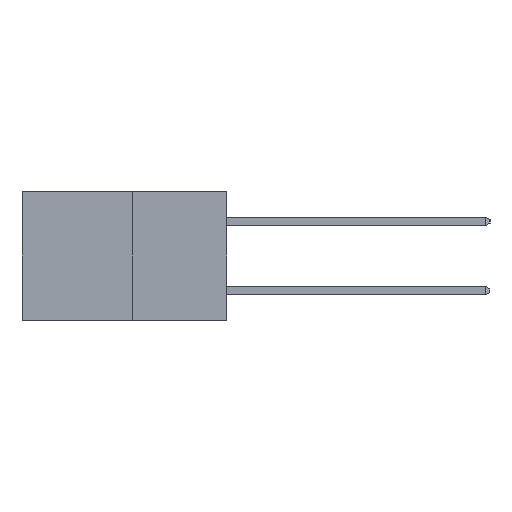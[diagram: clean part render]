
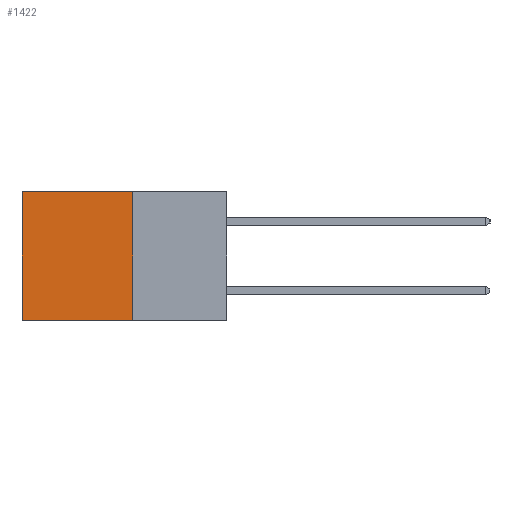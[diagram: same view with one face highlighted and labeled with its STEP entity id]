
A CAD part, left-side view. The second image highlights one B-rep face of the part: STEP entity #1422.
In plain terms, the highlighted planar face has unit normal (-1, 0, 0).
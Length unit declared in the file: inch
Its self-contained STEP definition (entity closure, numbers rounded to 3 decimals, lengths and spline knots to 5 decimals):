
#739 = DIRECTION ( 'NONE',  ( 0., 1., 0. ) ) ;
#784 = AXIS2_PLACEMENT_3D ( 'NONE', #6101, #7769, #3082 ) ;
#793 = CARTESIAN_POINT ( 'NONE',  ( 0.277, 0.59, -0.37 ) ) ;
#1271 = DIRECTION ( 'NONE',  ( 0., 1., 0. ) ) ;
#1422 = ADVANCED_FACE ( 'NONE', ( #7081 ), #3141, .F. ) ;
#1461 = DIRECTION ( 'NONE',  ( 0., 0., -1. ) ) ;
#1552 = CARTESIAN_POINT ( 'NONE',  ( 0.277, 0.27, -0.37 ) ) ;
#2052 = DIRECTION ( 'NONE',  ( 0., 0., -1. ) ) ;
#2088 = CARTESIAN_POINT ( 'NONE',  ( 0.277, 0.59, -0.37 ) ) ;
#2258 = CARTESIAN_POINT ( 'NONE',  ( 0.277, 0.27, 0. ) ) ;
#2461 = VERTEX_POINT ( 'NONE', #7559 ) ;
#2623 = VERTEX_POINT ( 'NONE', #793 ) ;
#2718 = VERTEX_POINT ( 'NONE', #5380 ) ;
#2826 = EDGE_CURVE ( 'NONE', #5962, #2461, #8480, .T. ) ;
#3020 = VECTOR ( 'NONE', #2052, 39.37008 ) ;
#3082 = DIRECTION ( 'NONE',  ( 0., 0., -1. ) ) ;
#3141 = PLANE ( 'NONE',  #784 ) ;
#3353 = LINE ( 'NONE', #5447, #5680 ) ;
#3740 = EDGE_CURVE ( 'NONE', #2461, #2623, #9834, .T. ) ;
#3789 = VECTOR ( 'NONE', #1271, 39.37008 ) ;
#5097 = LINE ( 'NONE', #2088, #3020 ) ;
#5380 = CARTESIAN_POINT ( 'NONE',  ( 0.277, 0.59, 0. ) ) ;
#5447 = CARTESIAN_POINT ( 'NONE',  ( 0.277, 0.27, 0. ) ) ;
#5590 = ORIENTED_EDGE ( 'NONE', *, *, #5999, .T. ) ;
#5680 = VECTOR ( 'NONE', #739, 39.37008 ) ;
#5773 = VECTOR ( 'NONE', #1461, 39.37008 ) ;
#5962 = VERTEX_POINT ( 'NONE', #2258 ) ;
#5999 = EDGE_CURVE ( 'NONE', #2718, #2623, #5097, .T. ) ;
#6101 = CARTESIAN_POINT ( 'NONE',  ( 0.277, 0.27, -0.37 ) ) ;
#7081 = FACE_OUTER_BOUND ( 'NONE', #7477, .T. ) ;
#7464 = EDGE_CURVE ( 'NONE', #5962, #2718, #3353, .T. ) ;
#7477 = EDGE_LOOP ( 'NONE', ( #5590, #7909, #8401, #9602 ) ) ;
#7559 = CARTESIAN_POINT ( 'NONE',  ( 0.277, 0.27, -0.37 ) ) ;
#7769 = DIRECTION ( 'NONE',  ( 1., 0., 0. ) ) ;
#7909 = ORIENTED_EDGE ( 'NONE', *, *, #3740, .F. ) ;
#8401 = ORIENTED_EDGE ( 'NONE', *, *, #2826, .F. ) ;
#8480 = LINE ( 'NONE', #1552, #5773 ) ;
#9602 = ORIENTED_EDGE ( 'NONE', *, *, #7464, .T. ) ;
#9834 = LINE ( 'NONE', #9942, #3789 ) ;
#9942 = CARTESIAN_POINT ( 'NONE',  ( 0.277, 0.27, -0.37 ) ) ;
